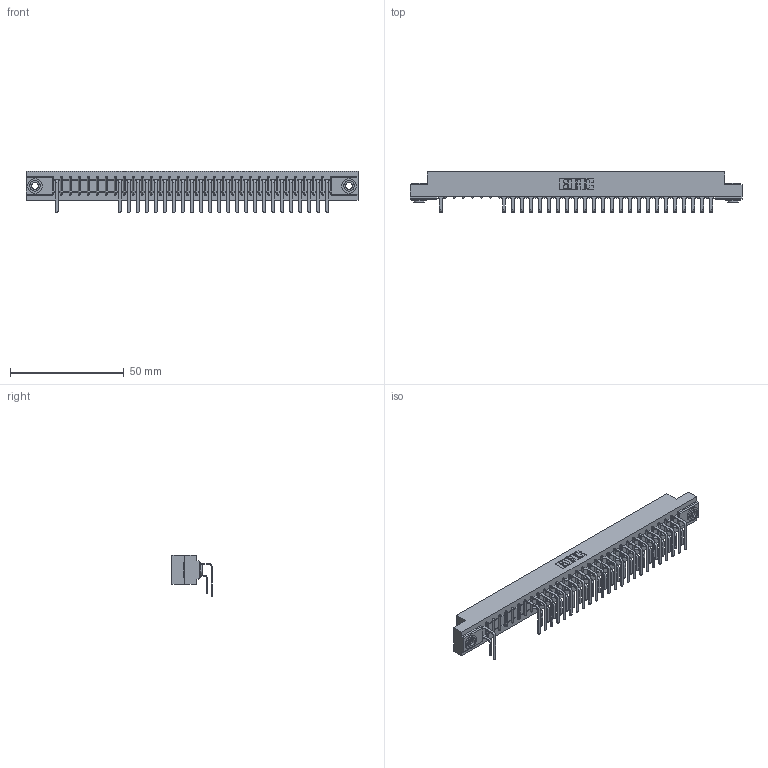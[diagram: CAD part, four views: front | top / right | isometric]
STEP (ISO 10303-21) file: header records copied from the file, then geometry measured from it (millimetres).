
FILE_DESCRIPTION (( 'STEP AP203' ), '1' );
FILE_NAME ('307-031-559-103.STEP', '2018-08-04T20:36:23', ( '' ), ( '' ), 'SwSTEP 2.0', 'SolidWorks 2016', '' );
FILE_SCHEMA (( 'CONFIG_CONTROL_DESIGN' ));
Length unit declared in the file: inch
Products named in the file (5): 307-290-001_559 - 2 (Single); 345-250-002_345-250-002-102; 307-031-559-103; 307 Part_.156 Dia Mounting Holes; 307-290-001_558 559 - 1 (Single)
Assembly tree (52 placements, depth 2):
  307-031-559-103
    307 Part_.156 Dia Mounting Holes
    307-290-001_558 559 - 1 (Single)  x24
    307-290-001_559 - 2 (Single)  x25
    345-250-002_345-250-002-102  x2
Bounding box: 145.85 x 17.69 x 18.07 mm (x, y, z)
Volume: 15483 mm3; surface area: 19143.9 mm2
Topology: 52 solids, 52 shells, 2782 faces, 7809 edges, 5050 vertices
Faces by surface type: plane 1789, cylinder 921, sphere 64, cone 8
Entity records: 31020 total; most frequent: CARTESIAN_POINT 5117, ORIENTED_EDGE 5074, DIRECTION 5017, EDGE_CURVE 2537, LINE 1933, VECTOR 1933, VERTEX_POINT 1642, AXIS2_PLACEMENT_3D 1542
